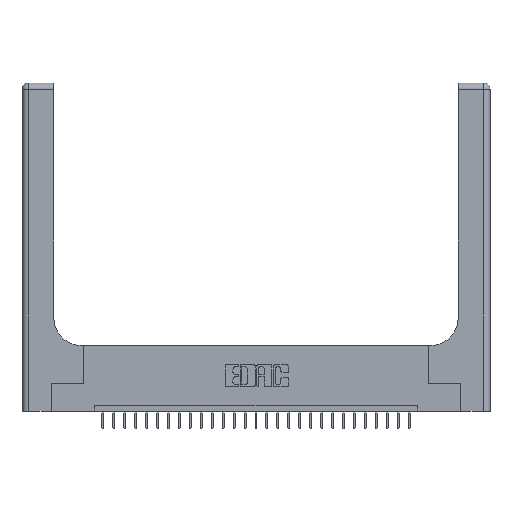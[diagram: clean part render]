
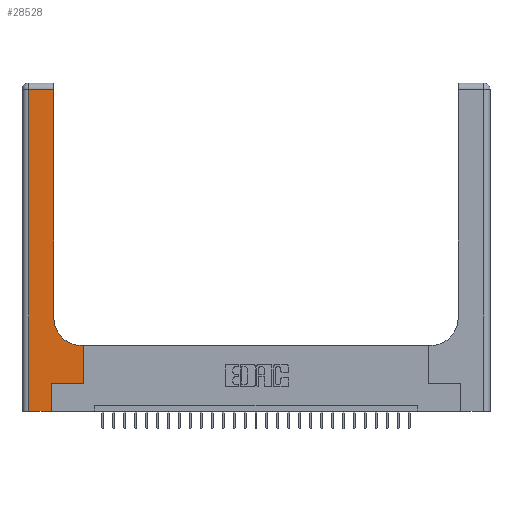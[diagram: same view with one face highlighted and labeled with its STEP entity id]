
A CAD part, top view. The second image highlights one B-rep face of the part: STEP entity #28528.
In plain terms, the highlighted planar face has unit normal (0, 0, 1).
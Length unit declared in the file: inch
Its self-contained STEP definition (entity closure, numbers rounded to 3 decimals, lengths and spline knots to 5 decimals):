
#369 = VERTEX_POINT ( 'NONE', #22483 ) ;
#438 = CARTESIAN_POINT ( 'NONE',  ( 0., 2.94, 0.37 ) ) ;
#745 = AXIS2_PLACEMENT_3D ( 'NONE', #21806, #3671, #21512 ) ;
#1349 = EDGE_CURVE ( 'NONE', #15266, #18151, #15314, .T. ) ;
#1893 = ORIENTED_EDGE ( 'NONE', *, *, #22968, .T. ) ;
#2201 = DIRECTION ( 'NONE',  ( 0., 1., 0. ) ) ;
#2213 = VECTOR ( 'NONE', #6435, 39.37008 ) ;
#2683 = DIRECTION ( 'NONE',  ( -1., 0., 0. ) ) ;
#2809 = VERTEX_POINT ( 'NONE', #12864 ) ;
#3243 = LINE ( 'NONE', #24308, #2213 ) ;
#3296 = CARTESIAN_POINT ( 'NONE',  ( 0.5585, 0.6, 0.37 ) ) ;
#3671 = DIRECTION ( 'NONE',  ( 0., 0., -1. ) ) ;
#4131 = EDGE_CURVE ( 'NONE', #20691, #15266, #4272, .T. ) ;
#4272 = LINE ( 'NONE', #10124, #9137 ) ;
#5062 = CARTESIAN_POINT ( 'NONE',  ( 0., 3., 0.37 ) ) ;
#5113 = ORIENTED_EDGE ( 'NONE', *, *, #7428, .T. ) ;
#5156 = DIRECTION ( 'NONE',  ( 0., 1., 0. ) ) ;
#5659 = DIRECTION ( 'NONE',  ( 0., -1., 0. ) ) ;
#5801 = EDGE_CURVE ( 'NONE', #18741, #369, #16773, .T. ) ;
#5841 = VECTOR ( 'NONE', #2201, 39.37008 ) ;
#6435 = DIRECTION ( 'NONE',  ( 0., 1., 0. ) ) ;
#6741 = AXIS2_PLACEMENT_3D ( 'NONE', #5062, #20975, #7596 ) ;
#6801 = LINE ( 'NONE', #16389, #16231 ) ;
#6805 = CARTESIAN_POINT ( 'NONE',  ( 0.5415, 0.6, 0.37 ) ) ;
#6833 = CARTESIAN_POINT ( 'NONE',  ( 0.5585, 0.25, 0.37 ) ) ;
#7174 = VECTOR ( 'NONE', #2683, 39.37008 ) ;
#7428 = EDGE_CURVE ( 'NONE', #18915, #18741, #22236, .T. ) ;
#7596 = DIRECTION ( 'NONE',  ( -1., 0., 0. ) ) ;
#8377 = EDGE_CURVE ( 'NONE', #17830, #11780, #6801, .T. ) ;
#8631 = CARTESIAN_POINT ( 'NONE',  ( 0.5585, 0.25, 0.37 ) ) ;
#8992 = CARTESIAN_POINT ( 'NONE',  ( 0.269, 0.25, 0.37 ) ) ;
#9137 = VECTOR ( 'NONE', #5659, 39.37008 ) ;
#10124 = CARTESIAN_POINT ( 'NONE',  ( 0.06, 3., 0.37 ) ) ;
#10418 = EDGE_CURVE ( 'NONE', #369, #2809, #16743, .T. ) ;
#11719 = DIRECTION ( 'NONE',  ( 1., 0., 0. ) ) ;
#11780 = VERTEX_POINT ( 'NONE', #6833 ) ;
#11783 = LINE ( 'NONE', #8631, #5841 ) ;
#12864 = CARTESIAN_POINT ( 'NONE',  ( 0.2915, 2.94, 0.37 ) ) ;
#13231 = VECTOR ( 'NONE', #28707, 39.37008 ) ;
#13994 = PLANE ( 'NONE',  #6741 ) ;
#14137 = DIRECTION ( 'NONE',  ( -1., 0., 0. ) ) ;
#14268 = VECTOR ( 'NONE', #5156, 39.37008 ) ;
#14748 = ORIENTED_EDGE ( 'NONE', *, *, #10418, .T. ) ;
#15266 = VERTEX_POINT ( 'NONE', #25816 ) ;
#15314 = LINE ( 'NONE', #28424, #13231 ) ;
#16061 = CARTESIAN_POINT ( 'NONE',  ( 0.2915, 3., 0.37 ) ) ;
#16075 = EDGE_CURVE ( 'NONE', #2809, #20691, #26032, .T. ) ;
#16213 = CARTESIAN_POINT ( 'NONE',  ( 0.2915, 0.6, 0.37 ) ) ;
#16231 = VECTOR ( 'NONE', #11719, 39.37008 ) ;
#16389 = CARTESIAN_POINT ( 'NONE',  ( 0.269, 0.25, 0.37 ) ) ;
#16743 = LINE ( 'NONE', #16061, #14268 ) ;
#16773 = CIRCLE ( 'NONE', #745, 0.25 ) ;
#17375 = VECTOR ( 'NONE', #14137, 39.37008 ) ;
#17830 = VERTEX_POINT ( 'NONE', #8992 ) ;
#18151 = VERTEX_POINT ( 'NONE', #22156 ) ;
#18711 = EDGE_CURVE ( 'NONE', #18151, #17830, #3243, .T. ) ;
#18741 = VERTEX_POINT ( 'NONE', #6805 ) ;
#18915 = VERTEX_POINT ( 'NONE', #3296 ) ;
#19291 = ORIENTED_EDGE ( 'NONE', *, *, #1349, .T. ) ;
#20691 = VERTEX_POINT ( 'NONE', #24822 ) ;
#20912 = FACE_OUTER_BOUND ( 'NONE', #22570, .T. ) ;
#20975 = DIRECTION ( 'NONE',  ( 0., 0., -1. ) ) ;
#21114 = ORIENTED_EDGE ( 'NONE', *, *, #16075, .T. ) ;
#21512 = DIRECTION ( 'NONE',  ( 1., 0., 0. ) ) ;
#21806 = CARTESIAN_POINT ( 'NONE',  ( 0.5415, 0.85, 0.37 ) ) ;
#22156 = CARTESIAN_POINT ( 'NONE',  ( 0.269, 0., 0.37 ) ) ;
#22236 = LINE ( 'NONE', #16213, #17375 ) ;
#22483 = CARTESIAN_POINT ( 'NONE',  ( 0.2915, 0.85, 0.37 ) ) ;
#22541 = ORIENTED_EDGE ( 'NONE', *, *, #4131, .T. ) ;
#22570 = EDGE_LOOP ( 'NONE', ( #14748, #21114, #22541, #19291, #25949, #28686, #1893, #5113, #27022 ) ) ;
#22968 = EDGE_CURVE ( 'NONE', #11780, #18915, #11783, .T. ) ;
#24308 = CARTESIAN_POINT ( 'NONE',  ( 0.269, 0., 0.37 ) ) ;
#24822 = CARTESIAN_POINT ( 'NONE',  ( 0.06, 2.94, 0.37 ) ) ;
#25816 = CARTESIAN_POINT ( 'NONE',  ( 0.06, 0., 0.37 ) ) ;
#25949 = ORIENTED_EDGE ( 'NONE', *, *, #18711, .T. ) ;
#26032 = LINE ( 'NONE', #438, #7174 ) ;
#27022 = ORIENTED_EDGE ( 'NONE', *, *, #5801, .T. ) ;
#28424 = CARTESIAN_POINT ( 'NONE',  ( 0., 0., 0.37 ) ) ;
#28528 = ADVANCED_FACE ( 'NONE', ( #20912 ), #13994, .F. ) ;
#28686 = ORIENTED_EDGE ( 'NONE', *, *, #8377, .T. ) ;
#28707 = DIRECTION ( 'NONE',  ( 1., 0., 0. ) ) ;
